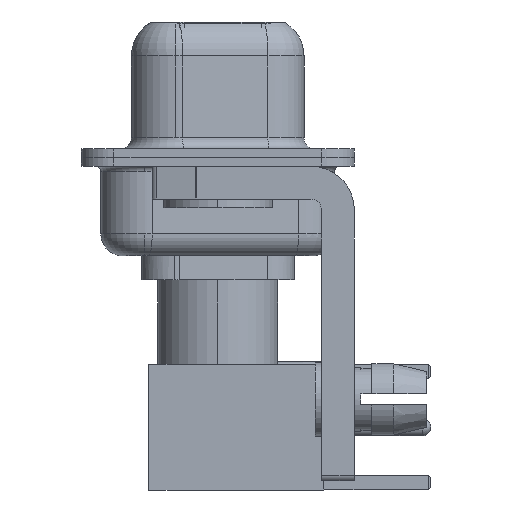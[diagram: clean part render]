
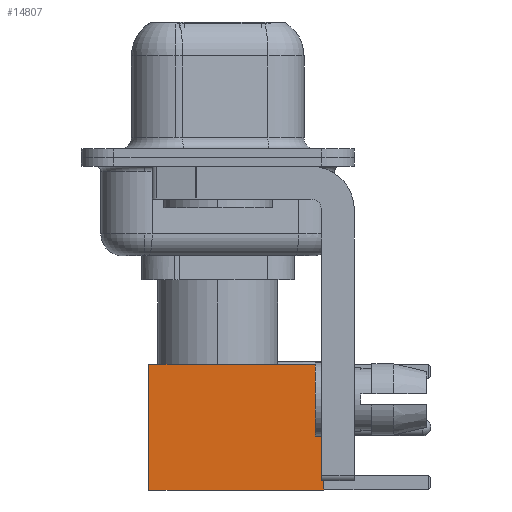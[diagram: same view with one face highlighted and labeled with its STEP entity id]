
A CAD part, left-side view. The second image highlights one B-rep face of the part: STEP entity #14807.
In plain terms, the highlighted face is planar.
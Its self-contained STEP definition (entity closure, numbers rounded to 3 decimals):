
#158 = DIRECTION ( 'NONE',  ( -1., 0., 0. ) ) ;
#1717 = CARTESIAN_POINT ( 'NONE',  ( -2.875, 2.875, 8. ) ) ;
#2168 = EDGE_CURVE ( 'NONE', #7524, #22589, #4998, .T. ) ;
#4263 = DIRECTION ( 'NONE',  ( 0., 0., -1. ) ) ;
#4834 = LINE ( 'NONE', #20919, #28862 ) ;
#4998 = LINE ( 'NONE', #12820, #26198 ) ;
#5907 = EDGE_LOOP ( 'NONE', ( #28811, #22607, #27865, #24198 ) ) ;
#7204 = VERTEX_POINT ( 'NONE', #1717 ) ;
#7372 = VECTOR ( 'NONE', #20478, 1000. ) ;
#7423 = EDGE_CURVE ( 'NONE', #7204, #22589, #4834, .T. ) ;
#7524 = VERTEX_POINT ( 'NONE', #19092 ) ;
#8309 = CARTESIAN_POINT ( 'NONE',  ( 2.875, 2.875, 8. ) ) ;
#11000 = CARTESIAN_POINT ( 'NONE',  ( -2.875, 2.875, 0. ) ) ;
#11613 = LINE ( 'NONE', #18454, #21041 ) ;
#12820 = CARTESIAN_POINT ( 'NONE',  ( 0., 2.875, 0. ) ) ;
#12855 = VERTEX_POINT ( 'NONE', #8309 ) ;
#14807 = ADVANCED_FACE ( 'NONE', ( #25879 ), #23921, .T. ) ;
#15924 = EDGE_CURVE ( 'NONE', #12855, #7524, #24402, .T. ) ;
#18454 = CARTESIAN_POINT ( 'NONE',  ( 0., 2.875, 8. ) ) ;
#18617 = DIRECTION ( 'NONE',  ( 0., 0., 1. ) ) ;
#19092 = CARTESIAN_POINT ( 'NONE',  ( 2.875, 2.875, 0. ) ) ;
#20478 = DIRECTION ( 'NONE',  ( 0., 0., -1. ) ) ;
#20919 = CARTESIAN_POINT ( 'NONE',  ( -2.875, 2.875, 0. ) ) ;
#21041 = VECTOR ( 'NONE', #158, 1000. ) ;
#21919 = DIRECTION ( 'NONE',  ( -1., 0., 0. ) ) ;
#22122 = CARTESIAN_POINT ( 'NONE',  ( 2.875, 2.875, 0. ) ) ;
#22396 = EDGE_CURVE ( 'NONE', #12855, #7204, #11613, .T. ) ;
#22589 = VERTEX_POINT ( 'NONE', #11000 ) ;
#22607 = ORIENTED_EDGE ( 'NONE', *, *, #2168, .T. ) ;
#23299 = CARTESIAN_POINT ( 'NONE',  ( 2.875, 2.875, 0. ) ) ;
#23891 = AXIS2_PLACEMENT_3D ( 'NONE', #23299, #27999, #18617 ) ;
#23921 = PLANE ( 'NONE',  #23891 ) ;
#24198 = ORIENTED_EDGE ( 'NONE', *, *, #22396, .F. ) ;
#24402 = LINE ( 'NONE', #22122, #7372 ) ;
#25879 = FACE_OUTER_BOUND ( 'NONE', #5907, .T. ) ;
#26198 = VECTOR ( 'NONE', #21919, 1000. ) ;
#27865 = ORIENTED_EDGE ( 'NONE', *, *, #7423, .F. ) ;
#27999 = DIRECTION ( 'NONE',  ( 0., 1., 0. ) ) ;
#28811 = ORIENTED_EDGE ( 'NONE', *, *, #15924, .T. ) ;
#28862 = VECTOR ( 'NONE', #4263, 1000. ) ;
